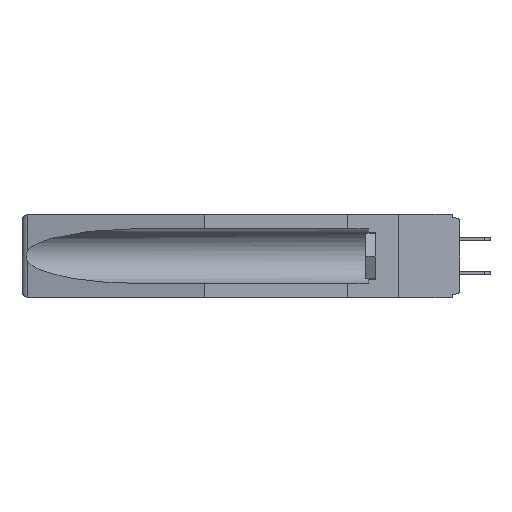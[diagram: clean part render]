
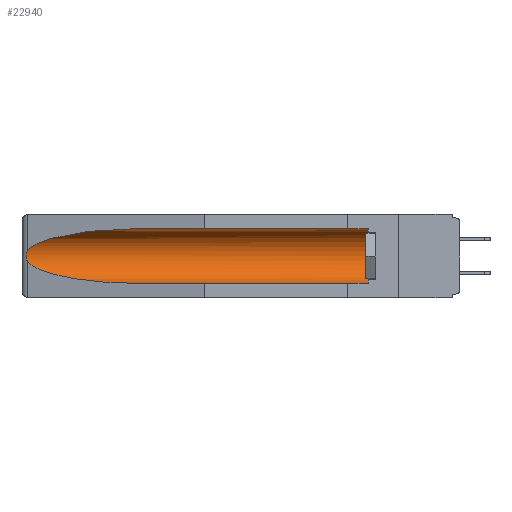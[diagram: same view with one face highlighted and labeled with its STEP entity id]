
A CAD part, left-side view. The second image highlights one B-rep face of the part: STEP entity #22940.
In plain terms, the highlighted cylindrical face has radius 2.857 mm (diameter 5.715 mm), a partial arc.
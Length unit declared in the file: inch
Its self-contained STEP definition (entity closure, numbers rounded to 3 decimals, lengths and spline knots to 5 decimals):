
#64 = EDGE_CURVE ( 'NONE', #13050, #9538, #4772, .T. ) ;
#171 = CARTESIAN_POINT ( 'NONE',  ( 0.25451, 1.48313, -0.24835 ) ) ;
#379 = CARTESIAN_POINT ( 'NONE',  ( 0.2673, 1.53269, -0.17917 ) ) ;
#1529 = CARTESIAN_POINT ( 'NONE',  ( 0.26654, 1.53092, -0.15636 ) ) ;
#1753 = DIRECTION ( 'NONE',  ( 0., -1., 0. ) ) ;
#1783 = VECTOR ( 'NONE', #13370, 39.37008 ) ;
#1841 = CARTESIAN_POINT ( 'NONE',  ( 0.21114, 1.30732, -0.059 ) ) ;
#2187 = EDGE_CURVE ( 'NONE', #15637, #25184, #17248, .T. ) ;
#2245 = CARTESIAN_POINT ( 'NONE',  ( 0.21114, 1.30732, -0.284 ) ) ;
#2306 = CARTESIAN_POINT ( 'NONE',  ( 0.26537, 1.52718, -0.14972 ) ) ;
#2336 = CARTESIAN_POINT ( 'NONE',  ( 0.155, 1.07973, -0.284 ) ) ;
#3735 = AXIS2_PLACEMENT_3D ( 'NONE', #15423, #1753, #11076 ) ;
#4089 = DIRECTION ( 'NONE',  ( 0., 1., 0. ) ) ;
#4457 = ORIENTED_EDGE ( 'NONE', *, *, #27289, .T. ) ;
#4772 = CIRCLE ( 'NONE', #3735, 0.1125 ) ;
#6668 = CYLINDRICAL_SURFACE ( 'NONE', #14138, 0.1125 ) ;
#7885 = LINE ( 'NONE', #20460, #1783 ) ;
#8449 = LINE ( 'NONE', #26964, #27019 ) ;
#9538 = VERTEX_POINT ( 'NONE', #22868 ) ;
#9675 = CARTESIAN_POINT ( 'NONE',  ( 0.26597, 1.5296, -0.19026 ) ) ;
#10471 = ORIENTED_EDGE ( 'NONE', *, *, #19921, .T. ) ;
#10825 = ORIENTED_EDGE ( 'NONE', *, *, #64, .T. ) ;
#10910 = CARTESIAN_POINT ( 'NONE',  ( 0.155, 1.07973, -0.059 ) ) ;
#11076 = DIRECTION ( 'NONE',  ( 0., 0., 1. ) ) ;
#11236 = DIRECTION ( 'NONE',  ( 0., 0., 1. ) ) ;
#12958 = EDGE_CURVE ( 'NONE', #22219, #15637, #18561, .T. ) ;
#13050 = VERTEX_POINT ( 'NONE', #22620 ) ;
#13370 = DIRECTION ( 'NONE',  ( 0., 1., 0. ) ) ;
#13426 = CARTESIAN_POINT ( 'NONE',  ( 0.25451, 1.48313, -0.09465 ) ) ;
#13781 =( BOUNDED_CURVE ( )  B_SPLINE_CURVE ( 3, ( #16027, #171, #2245, #2336 ),
 .UNSPECIFIED., .F., .F. ) 
 B_SPLINE_CURVE_WITH_KNOTS ( ( 4, 4 ),
 ( 0.1948, 1.5708 ),
 .UNSPECIFIED. ) 
 CURVE ( )  GEOMETRIC_REPRESENTATION_ITEM ( )  RATIONAL_B_SPLINE_CURVE ( ( 1., 0.848, 0.848, 1. ) ) 
 REPRESENTATION_ITEM ( '' )  );
#14138 = AXIS2_PLACEMENT_3D ( 'NONE', #27396, #20315, #11236 ) ;
#15423 = CARTESIAN_POINT ( 'NONE',  ( 0.155, 0.126, -0.1715 ) ) ;
#15637 = VERTEX_POINT ( 'NONE', #2306 ) ;
#16027 = CARTESIAN_POINT ( 'NONE',  ( 0.26537, 1.52718, -0.19328 ) ) ;
#16503 = EDGE_CURVE ( 'NONE', #13050, #27539, #8449, .T. ) ;
#16640 = CARTESIAN_POINT ( 'NONE',  ( 0.26655, 1.53094, -0.18657 ) ) ;
#17248 = B_SPLINE_CURVE_WITH_KNOTS ( 'NONE', 3,
 ( #25110, #28659, #1529, #27927, #25786, #23543, #379, #16640, #9675, #21205 ),
 .UNSPECIFIED., .F., .F.,
 ( 4, 2, 2, 2, 4 ),
 ( 0., 0.00029, 0.00058, 0.00087, 0.00117 ),
 .UNSPECIFIED. ) ;
#18561 =( BOUNDED_CURVE ( )  B_SPLINE_CURVE ( 3, ( #20019, #1841, #13426, #29388 ),
 .UNSPECIFIED., .F., .T. ) 
 B_SPLINE_CURVE_WITH_KNOTS ( ( 4, 4 ),
 ( 4.71239, 6.08839 ),
 .UNSPECIFIED. ) 
 CURVE ( )  GEOMETRIC_REPRESENTATION_ITEM ( )  RATIONAL_B_SPLINE_CURVE ( ( 1., 0.848, 0.848, 1. ) ) 
 REPRESENTATION_ITEM ( '' )  );
#19921 = EDGE_CURVE ( 'NONE', #25184, #27539, #13781, .T. ) ;
#20019 = CARTESIAN_POINT ( 'NONE',  ( 0.155, 1.07973, -0.059 ) ) ;
#20315 = DIRECTION ( 'NONE',  ( 0., 1., 0. ) ) ;
#20460 = CARTESIAN_POINT ( 'NONE',  ( 0.155, -0.30754, -0.059 ) ) ;
#21149 = ORIENTED_EDGE ( 'NONE', *, *, #2187, .T. ) ;
#21205 = CARTESIAN_POINT ( 'NONE',  ( 0.26537, 1.52718, -0.19328 ) ) ;
#21237 = FACE_OUTER_BOUND ( 'NONE', #23636, .T. ) ;
#21746 = CARTESIAN_POINT ( 'NONE',  ( 0.26537, 1.52718, -0.19328 ) ) ;
#22219 = VERTEX_POINT ( 'NONE', #10910 ) ;
#22620 = CARTESIAN_POINT ( 'NONE',  ( 0.155, 0.126, -0.284 ) ) ;
#22778 = ORIENTED_EDGE ( 'NONE', *, *, #12958, .T. ) ;
#22868 = CARTESIAN_POINT ( 'NONE',  ( 0.155, 0.126, -0.059 ) ) ;
#22940 = ADVANCED_FACE ( 'NONE', ( #21237 ), #6668, .F. ) ;
#23543 = CARTESIAN_POINT ( 'NONE',  ( 0.2675, 1.53308, -0.17534 ) ) ;
#23636 = EDGE_LOOP ( 'NONE', ( #22778, #21149, #10471, #24091, #10825, #4457 ) ) ;
#24091 = ORIENTED_EDGE ( 'NONE', *, *, #16503, .F. ) ;
#25110 = CARTESIAN_POINT ( 'NONE',  ( 0.26537, 1.52718, -0.14972 ) ) ;
#25184 = VERTEX_POINT ( 'NONE', #21746 ) ;
#25786 = CARTESIAN_POINT ( 'NONE',  ( 0.2675, 1.53308, -0.16763 ) ) ;
#26964 = CARTESIAN_POINT ( 'NONE',  ( 0.155, -0.30754, -0.284 ) ) ;
#27019 = VECTOR ( 'NONE', #4089, 39.37008 ) ;
#27289 = EDGE_CURVE ( 'NONE', #9538, #22219, #7885, .T. ) ;
#27396 = CARTESIAN_POINT ( 'NONE',  ( 0.155, -0.30754, -0.1715 ) ) ;
#27539 = VERTEX_POINT ( 'NONE', #28033 ) ;
#27927 = CARTESIAN_POINT ( 'NONE',  ( 0.2673, 1.5327, -0.16383 ) ) ;
#28033 = CARTESIAN_POINT ( 'NONE',  ( 0.155, 1.07973, -0.284 ) ) ;
#28659 = CARTESIAN_POINT ( 'NONE',  ( 0.26597, 1.52961, -0.15275 ) ) ;
#29388 = CARTESIAN_POINT ( 'NONE',  ( 0.26537, 1.52718, -0.14972 ) ) ;
